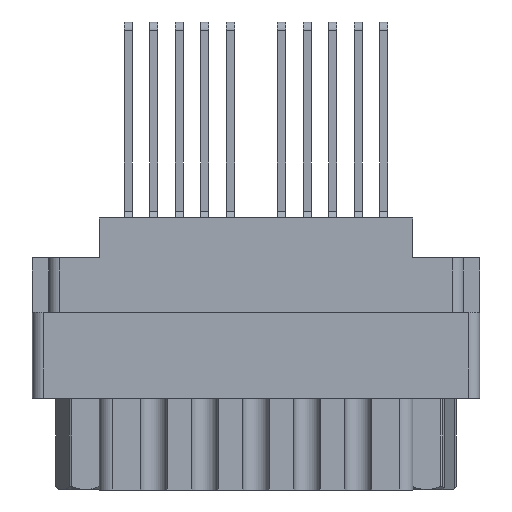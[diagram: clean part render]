
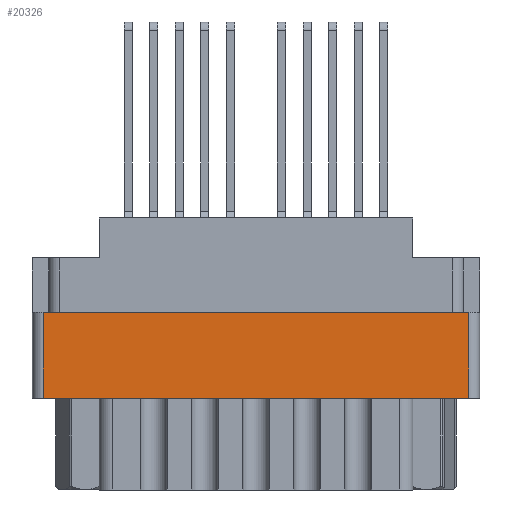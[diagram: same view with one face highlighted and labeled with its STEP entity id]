
A CAD part, front view. The second image highlights one B-rep face of the part: STEP entity #20326.
In plain terms, the highlighted planar face has unit normal (0, -1, 0).
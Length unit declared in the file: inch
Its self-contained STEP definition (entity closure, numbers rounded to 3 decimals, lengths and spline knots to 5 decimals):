
#169 = CARTESIAN_POINT ( 'NONE',  ( 0.624, -0.343, -0.529 ) ) ;
#657 = DIRECTION ( 'NONE',  ( 0., 0., 1. ) ) ;
#736 = VECTOR ( 'NONE', #23037, 39.37008 ) ;
#1446 = CARTESIAN_POINT ( 'NONE',  ( -0.624, -0.343, -0.277 ) ) ;
#1646 = EDGE_CURVE ( 'NONE', #21306, #18018, #14568, .T. ) ;
#1794 = EDGE_CURVE ( 'NONE', #34673, #2948, #4704, .T. ) ;
#2948 = VERTEX_POINT ( 'NONE', #27327 ) ;
#3167 = VECTOR ( 'NONE', #12699, 39.37008 ) ;
#4688 = DIRECTION ( 'NONE',  ( 0., -1., 0. ) ) ;
#4704 = LINE ( 'NONE', #18249, #28374 ) ;
#10208 = CARTESIAN_POINT ( 'NONE',  ( -0.656, -0.343, -0.798 ) ) ;
#11590 = DIRECTION ( 'NONE',  ( 0., 0., -1. ) ) ;
#12699 = DIRECTION ( 'NONE',  ( 1., 0., 0. ) ) ;
#14568 = LINE ( 'NONE', #25946, #20842 ) ;
#14736 = CARTESIAN_POINT ( 'NONE',  ( 0., -0.343, -0.529 ) ) ;
#18018 = VERTEX_POINT ( 'NONE', #24589 ) ;
#18249 = CARTESIAN_POINT ( 'NONE',  ( 0.624, -0.343, -0.798 ) ) ;
#18986 = PLANE ( 'NONE',  #29644 ) ;
#20326 = ADVANCED_FACE ( 'NONE', ( #30794 ), #18986, .T. ) ;
#20609 = ORIENTED_EDGE ( 'NONE', *, *, #1646, .T. ) ;
#20842 = VECTOR ( 'NONE', #11590, 39.37008 ) ;
#21110 = CARTESIAN_POINT ( 'NONE',  ( 0., -0.343, -0.277 ) ) ;
#21306 = VERTEX_POINT ( 'NONE', #1446 ) ;
#23037 = DIRECTION ( 'NONE',  ( -1., 0., 0. ) ) ;
#24589 = CARTESIAN_POINT ( 'NONE',  ( -0.624, -0.343, -0.529 ) ) ;
#25139 = EDGE_CURVE ( 'NONE', #21306, #2948, #30007, .T. ) ;
#25175 = ORIENTED_EDGE ( 'NONE', *, *, #1794, .T. ) ;
#25946 = CARTESIAN_POINT ( 'NONE',  ( -0.624, -0.343, -0.798 ) ) ;
#27327 = CARTESIAN_POINT ( 'NONE',  ( 0.624, -0.343, -0.277 ) ) ;
#27573 = LINE ( 'NONE', #14736, #736 ) ;
#27750 = EDGE_CURVE ( 'NONE', #34673, #18018, #27573, .T. ) ;
#28374 = VECTOR ( 'NONE', #657, 39.37008 ) ;
#29644 = AXIS2_PLACEMENT_3D ( 'NONE', #10208, #4688, #35867 ) ;
#30007 = LINE ( 'NONE', #21110, #3167 ) ;
#30794 = FACE_OUTER_BOUND ( 'NONE', #31779, .T. ) ;
#31215 = ORIENTED_EDGE ( 'NONE', *, *, #27750, .F. ) ;
#31779 = EDGE_LOOP ( 'NONE', ( #35464, #20609, #31215, #25175 ) ) ;
#34673 = VERTEX_POINT ( 'NONE', #169 ) ;
#35464 = ORIENTED_EDGE ( 'NONE', *, *, #25139, .F. ) ;
#35867 = DIRECTION ( 'NONE',  ( 0., 0., -1. ) ) ;
